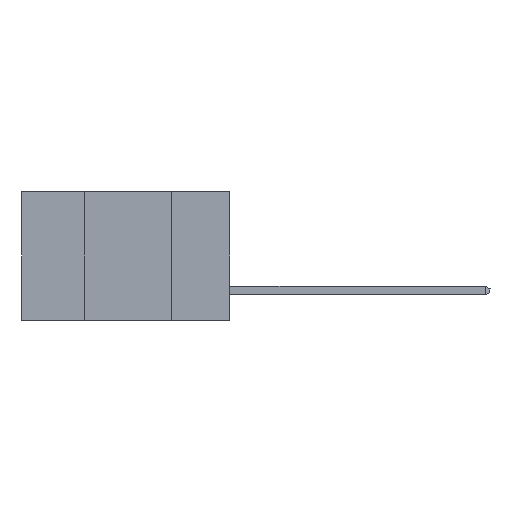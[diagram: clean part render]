
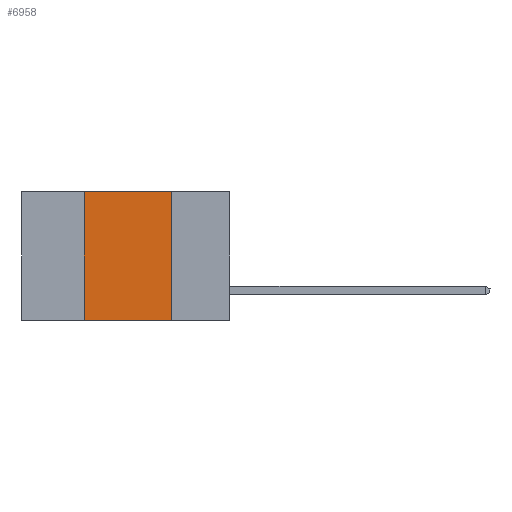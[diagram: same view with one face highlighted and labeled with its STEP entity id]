
A CAD part, left-side view. The second image highlights one B-rep face of the part: STEP entity #6958.
In plain terms, the highlighted planar face has unit normal (-1, 0, 0).
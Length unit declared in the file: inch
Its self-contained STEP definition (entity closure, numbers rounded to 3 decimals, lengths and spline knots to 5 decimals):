
#303 = VERTEX_POINT ( 'NONE', #19899 ) ;
#613 = CARTESIAN_POINT ( 'NONE',  ( 0., 0.17, -0.37 ) ) ;
#634 = VECTOR ( 'NONE', #6374, 39.37008 ) ;
#2401 = VECTOR ( 'NONE', #2799, 39.37008 ) ;
#2577 = CARTESIAN_POINT ( 'NONE',  ( 0., 0.42, -0.37 ) ) ;
#2799 = DIRECTION ( 'NONE',  ( 0., 0., -1. ) ) ;
#3092 = ORIENTED_EDGE ( 'NONE', *, *, #17313, .F. ) ;
#3978 = VECTOR ( 'NONE', #10062, 39.37008 ) ;
#4176 = EDGE_LOOP ( 'NONE', ( #17815, #5498, #3092, #10778 ) ) ;
#4455 = CARTESIAN_POINT ( 'NONE',  ( 0., 0.6, -0.37 ) ) ;
#4930 = DIRECTION ( 'NONE',  ( 0., 0., -1. ) ) ;
#5354 = VERTEX_POINT ( 'NONE', #16766 ) ;
#5498 = ORIENTED_EDGE ( 'NONE', *, *, #14033, .F. ) ;
#5670 = AXIS2_PLACEMENT_3D ( 'NONE', #6631, #12288, #4930 ) ;
#6043 = LINE ( 'NONE', #4455, #22398 ) ;
#6374 = DIRECTION ( 'NONE',  ( 0., -1., 0. ) ) ;
#6631 = CARTESIAN_POINT ( 'NONE',  ( 0., 0.6, 0. ) ) ;
#6958 = ADVANCED_FACE ( 'NONE', ( #17673 ), #21586, .F. ) ;
#9603 = DIRECTION ( 'NONE',  ( 0., -1., 0. ) ) ;
#10062 = DIRECTION ( 'NONE',  ( 0., 0., 1. ) ) ;
#10291 = LINE ( 'NONE', #2577, #3978 ) ;
#10778 = ORIENTED_EDGE ( 'NONE', *, *, #11884, .T. ) ;
#11766 = CARTESIAN_POINT ( 'NONE',  ( 0., 0.6, 0. ) ) ;
#11884 = EDGE_CURVE ( 'NONE', #13267, #5354, #6043, .T. ) ;
#12288 = DIRECTION ( 'NONE',  ( 1., 0., 0. ) ) ;
#13267 = VERTEX_POINT ( 'NONE', #16076 ) ;
#14033 = EDGE_CURVE ( 'NONE', #303, #18134, #21207, .T. ) ;
#15797 = LINE ( 'NONE', #613, #2401 ) ;
#16076 = CARTESIAN_POINT ( 'NONE',  ( 0., 0.42, -0.37 ) ) ;
#16766 = CARTESIAN_POINT ( 'NONE',  ( 0., 0.17, -0.37 ) ) ;
#17313 = EDGE_CURVE ( 'NONE', #13267, #303, #10291, .T. ) ;
#17673 = FACE_OUTER_BOUND ( 'NONE', #4176, .T. ) ;
#17815 = ORIENTED_EDGE ( 'NONE', *, *, #23060, .F. ) ;
#18134 = VERTEX_POINT ( 'NONE', #21837 ) ;
#19899 = CARTESIAN_POINT ( 'NONE',  ( 0., 0.42, 0. ) ) ;
#21207 = LINE ( 'NONE', #11766, #634 ) ;
#21586 = PLANE ( 'NONE',  #5670 ) ;
#21837 = CARTESIAN_POINT ( 'NONE',  ( 0., 0.17, 0. ) ) ;
#22398 = VECTOR ( 'NONE', #9603, 39.37008 ) ;
#23060 = EDGE_CURVE ( 'NONE', #18134, #5354, #15797, .T. ) ;
